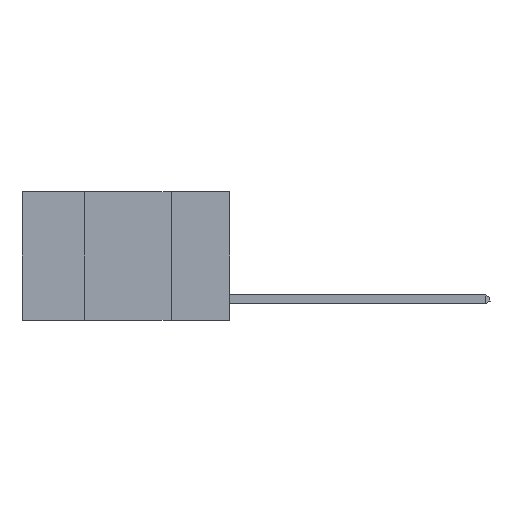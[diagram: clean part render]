
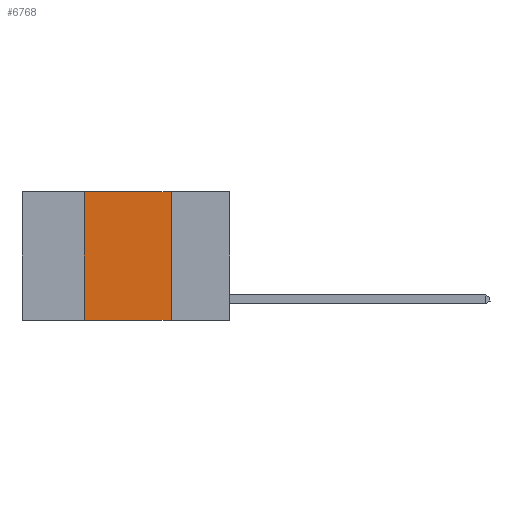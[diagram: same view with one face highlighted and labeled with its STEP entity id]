
A CAD part, left-side view. The second image highlights one B-rep face of the part: STEP entity #6768.
In plain terms, the highlighted planar face has unit normal (-1, 0, 0).
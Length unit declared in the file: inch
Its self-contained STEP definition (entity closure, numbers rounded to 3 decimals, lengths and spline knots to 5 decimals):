
#428 = CARTESIAN_POINT ( 'NONE',  ( 0., 0.6, 0. ) ) ;
#600 = EDGE_CURVE ( 'NONE', #13556, #11263, #1008, .T. ) ;
#882 = CARTESIAN_POINT ( 'NONE',  ( 0., 0.17, 0. ) ) ;
#1008 = LINE ( 'NONE', #11509, #9434 ) ;
#1168 = CARTESIAN_POINT ( 'NONE',  ( 0., 0.17, -0.37 ) ) ;
#2609 = DIRECTION ( 'NONE',  ( 0., 0., -1. ) ) ;
#3187 = AXIS2_PLACEMENT_3D ( 'NONE', #428, #9226, #2609 ) ;
#3731 = CARTESIAN_POINT ( 'NONE',  ( 0., 0.6, -0.37 ) ) ;
#4009 = VECTOR ( 'NONE', #6618, 39.37008 ) ;
#5083 = CARTESIAN_POINT ( 'NONE',  ( 0., 0.42, -0.37 ) ) ;
#5270 = ORIENTED_EDGE ( 'NONE', *, *, #13961, .T. ) ;
#6618 = DIRECTION ( 'NONE',  ( 0., -1., 0. ) ) ;
#6768 = ADVANCED_FACE ( 'NONE', ( #10064 ), #8147, .F. ) ;
#6896 = CARTESIAN_POINT ( 'NONE',  ( 0., 0.17, 0. ) ) ;
#7930 = DIRECTION ( 'NONE',  ( 0., 0., -1. ) ) ;
#8003 = LINE ( 'NONE', #3731, #13982 ) ;
#8147 = PLANE ( 'NONE',  #3187 ) ;
#8188 = VECTOR ( 'NONE', #7930, 39.37008 ) ;
#8531 = EDGE_CURVE ( 'NONE', #11263, #9083, #12338, .T. ) ;
#9083 = VERTEX_POINT ( 'NONE', #882 ) ;
#9226 = DIRECTION ( 'NONE',  ( 1., 0., 0. ) ) ;
#9255 = VERTEX_POINT ( 'NONE', #1168 ) ;
#9434 = VECTOR ( 'NONE', #11201, 39.37008 ) ;
#10064 = FACE_OUTER_BOUND ( 'NONE', #12227, .T. ) ;
#10209 = ORIENTED_EDGE ( 'NONE', *, *, #13236, .F. ) ;
#10280 = CARTESIAN_POINT ( 'NONE',  ( 0., 0.42, 0. ) ) ;
#10717 = ORIENTED_EDGE ( 'NONE', *, *, #600, .F. ) ;
#11201 = DIRECTION ( 'NONE',  ( 0., 0., 1. ) ) ;
#11263 = VERTEX_POINT ( 'NONE', #10280 ) ;
#11374 = DIRECTION ( 'NONE',  ( 0., -1., 0. ) ) ;
#11509 = CARTESIAN_POINT ( 'NONE',  ( 0., 0.42, 0. ) ) ;
#12227 = EDGE_LOOP ( 'NONE', ( #10209, #13159, #10717, #5270 ) ) ;
#12338 = LINE ( 'NONE', #13011, #4009 ) ;
#13011 = CARTESIAN_POINT ( 'NONE',  ( 0., 0.6, 0. ) ) ;
#13159 = ORIENTED_EDGE ( 'NONE', *, *, #8531, .F. ) ;
#13236 = EDGE_CURVE ( 'NONE', #9083, #9255, #13834, .T. ) ;
#13556 = VERTEX_POINT ( 'NONE', #5083 ) ;
#13834 = LINE ( 'NONE', #6896, #8188 ) ;
#13961 = EDGE_CURVE ( 'NONE', #13556, #9255, #8003, .T. ) ;
#13982 = VECTOR ( 'NONE', #11374, 39.37008 ) ;
